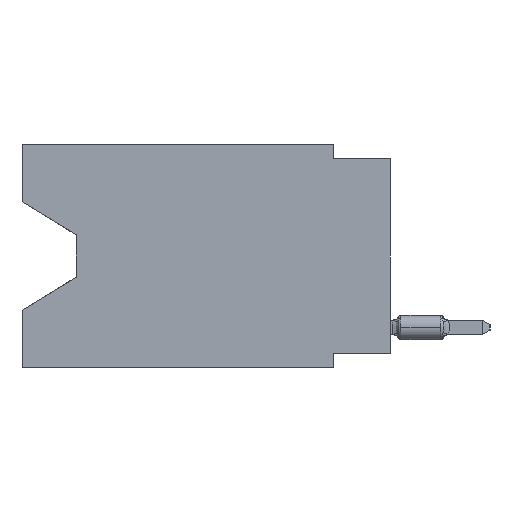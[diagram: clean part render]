
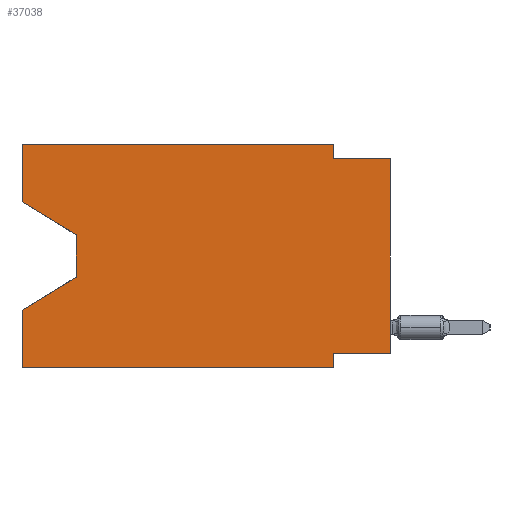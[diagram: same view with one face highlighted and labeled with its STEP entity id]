
A CAD part, left-side view. The second image highlights one B-rep face of the part: STEP entity #37038.
In plain terms, the highlighted planar face has unit normal (-1, 0, 0).
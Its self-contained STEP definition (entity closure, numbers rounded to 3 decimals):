
#512 = ORIENTED_EDGE ( 'NONE', *, *, #45183, .F. ) ;
#1542 = VERTEX_POINT ( 'NONE', #19705 ) ;
#1702 = ORIENTED_EDGE ( 'NONE', *, *, #9855, .F. ) ;
#1965 = DIRECTION ( 'NONE',  ( 0., -1., 0. ) ) ;
#3169 = LINE ( 'NONE', #44789, #12283 ) ;
#3433 = LINE ( 'NONE', #13735, #21825 ) ;
#4219 = EDGE_CURVE ( 'NONE', #1542, #48307, #7832, .T. ) ;
#4228 = CARTESIAN_POINT ( 'NONE',  ( 0., 16.383, -7.36 ) ) ;
#4435 = DIRECTION ( 'NONE',  ( 0., 0., -1. ) ) ;
#4763 = DIRECTION ( 'NONE',  ( 0., 0., -1. ) ) ;
#4885 = DIRECTION ( 'NONE',  ( 0., 0., -1. ) ) ;
#5386 = LINE ( 'NONE', #24705, #18495 ) ;
#5773 = LINE ( 'NONE', #24849, #22606 ) ;
#7021 = CARTESIAN_POINT ( 'NONE',  ( 0., 16.383, 0. ) ) ;
#7832 = LINE ( 'NONE', #16144, #19713 ) ;
#8362 = ORIENTED_EDGE ( 'NONE', *, *, #4219, .T. ) ;
#8756 = VERTEX_POINT ( 'NONE', #20245 ) ;
#9578 = EDGE_CURVE ( 'NONE', #43491, #15441, #5386, .T. ) ;
#9803 = EDGE_CURVE ( 'NONE', #30749, #11669, #10749, .T. ) ;
#9855 = EDGE_CURVE ( 'NONE', #47632, #23300, #3169, .T. ) ;
#10117 = DIRECTION ( 'NONE',  ( 0., -1., 0. ) ) ;
#10161 = EDGE_CURVE ( 'NONE', #8756, #43491, #21700, .T. ) ;
#10749 = LINE ( 'NONE', #17623, #23167 ) ;
#10930 = DIRECTION ( 'NONE',  ( 0., 0., -1. ) ) ;
#11669 = VERTEX_POINT ( 'NONE', #22764 ) ;
#12283 = VECTOR ( 'NONE', #26646, 1000. ) ;
#12544 = ORIENTED_EDGE ( 'NONE', *, *, #10161, .F. ) ;
#13652 = DIRECTION ( 'NONE',  ( 0., 0., 1. ) ) ;
#13709 = CARTESIAN_POINT ( 'NONE',  ( 0., 2.54, -9.271 ) ) ;
#13713 = EDGE_CURVE ( 'NONE', #15441, #32697, #48150, .T. ) ;
#13735 = CARTESIAN_POINT ( 'NONE',  ( 0., 0., -0.635 ) ) ;
#14557 = CARTESIAN_POINT ( 'NONE',  ( 0., 2.54, -9.906 ) ) ;
#14964 = CARTESIAN_POINT ( 'NONE',  ( 0., 0., -9.271 ) ) ;
#15086 = ORIENTED_EDGE ( 'NONE', *, *, #27840, .F. ) ;
#15441 = VERTEX_POINT ( 'NONE', #37149 ) ;
#15466 = FACE_OUTER_BOUND ( 'NONE', #23520, .T. ) ;
#15737 = LINE ( 'NONE', #30898, #34884 ) ;
#16144 = CARTESIAN_POINT ( 'NONE',  ( 0., 13.97, -4.013 ) ) ;
#16785 = AXIS2_PLACEMENT_3D ( 'NONE', #23030, #37999, #4435 ) ;
#17461 = VECTOR ( 'NONE', #34531, 1000. ) ;
#17623 = CARTESIAN_POINT ( 'NONE',  ( 0., 0., 0. ) ) ;
#17959 = ORIENTED_EDGE ( 'NONE', *, *, #21865, .F. ) ;
#18318 = CARTESIAN_POINT ( 'NONE',  ( 0., 2.54, -0.635 ) ) ;
#18495 = VECTOR ( 'NONE', #1965, 1000. ) ;
#19705 = CARTESIAN_POINT ( 'NONE',  ( 0., 13.97, -4.013 ) ) ;
#19713 = VECTOR ( 'NONE', #4885, 1000. ) ;
#20245 = CARTESIAN_POINT ( 'NONE',  ( 0., 16.383, -2.546 ) ) ;
#21497 = EDGE_CURVE ( 'NONE', #48307, #23300, #5773, .T. ) ;
#21700 = LINE ( 'NONE', #7021, #27119 ) ;
#21825 = VECTOR ( 'NONE', #47523, 1000. ) ;
#21865 = EDGE_CURVE ( 'NONE', #32697, #11669, #3433, .T. ) ;
#22606 = VECTOR ( 'NONE', #28757, 1000. ) ;
#22764 = CARTESIAN_POINT ( 'NONE',  ( 0., 0., -0.635 ) ) ;
#23030 = CARTESIAN_POINT ( 'NONE',  ( 0., 16.383, 0. ) ) ;
#23167 = VECTOR ( 'NONE', #40639, 1000. ) ;
#23300 = VERTEX_POINT ( 'NONE', #4228 ) ;
#23520 = EDGE_LOOP ( 'NONE', ( #45576, #8362, #45313, #1702, #41308, #512, #15086, #37245, #17959, #30543, #41993, #12544 ) ) ;
#23933 = LINE ( 'NONE', #42588, #17461 ) ;
#24389 = VERTEX_POINT ( 'NONE', #14557 ) ;
#24705 = CARTESIAN_POINT ( 'NONE',  ( 0., 16.383, 0. ) ) ;
#24849 = CARTESIAN_POINT ( 'NONE',  ( 0., 13.97, -5.893 ) ) ;
#26548 = EDGE_CURVE ( 'NONE', #8756, #1542, #23933, .T. ) ;
#26646 = DIRECTION ( 'NONE',  ( 0., 0., 1. ) ) ;
#26713 = PLANE ( 'NONE',  #16785 ) ;
#27119 = VECTOR ( 'NONE', #13652, 1000. ) ;
#27840 = EDGE_CURVE ( 'NONE', #30749, #31076, #15737, .T. ) ;
#28339 = CARTESIAN_POINT ( 'NONE',  ( 0., 13.97, -5.893 ) ) ;
#28757 = DIRECTION ( 'NONE',  ( 0., 0.855, -0.519 ) ) ;
#30543 = ORIENTED_EDGE ( 'NONE', *, *, #13713, .F. ) ;
#30749 = VERTEX_POINT ( 'NONE', #14964 ) ;
#30898 = CARTESIAN_POINT ( 'NONE',  ( 0., 0., -9.271 ) ) ;
#30948 = CARTESIAN_POINT ( 'NONE',  ( 0., 2.54, -9.906 ) ) ;
#31076 = VERTEX_POINT ( 'NONE', #13709 ) ;
#31426 = LINE ( 'NONE', #30948, #43567 ) ;
#32697 = VERTEX_POINT ( 'NONE', #18318 ) ;
#34531 = DIRECTION ( 'NONE',  ( 0., -0.855, -0.519 ) ) ;
#34591 = DIRECTION ( 'NONE',  ( 0., 1., 0. ) ) ;
#34884 = VECTOR ( 'NONE', #34591, 1000. ) ;
#35655 = VECTOR ( 'NONE', #10117, 1000. ) ;
#36087 = LINE ( 'NONE', #36325, #35655 ) ;
#36325 = CARTESIAN_POINT ( 'NONE',  ( 0., 16.383, -9.906 ) ) ;
#37038 = ADVANCED_FACE ( 'NONE', ( #15466 ), #26713, .F. ) ;
#37149 = CARTESIAN_POINT ( 'NONE',  ( 0., 2.54, 0. ) ) ;
#37162 = CARTESIAN_POINT ( 'NONE',  ( 0., 16.383, 0. ) ) ;
#37245 = ORIENTED_EDGE ( 'NONE', *, *, #9803, .T. ) ;
#37999 = DIRECTION ( 'NONE',  ( 1., 0., 0. ) ) ;
#40062 = CARTESIAN_POINT ( 'NONE',  ( 0., 16.383, -9.906 ) ) ;
#40639 = DIRECTION ( 'NONE',  ( 0., 0., 1. ) ) ;
#41308 = ORIENTED_EDGE ( 'NONE', *, *, #45413, .T. ) ;
#41993 = ORIENTED_EDGE ( 'NONE', *, *, #9578, .F. ) ;
#42588 = CARTESIAN_POINT ( 'NONE',  ( 0., 16.383, -2.546 ) ) ;
#43491 = VERTEX_POINT ( 'NONE', #37162 ) ;
#43567 = VECTOR ( 'NONE', #4763, 1000. ) ;
#44479 = CARTESIAN_POINT ( 'NONE',  ( 0., 2.54, 0. ) ) ;
#44789 = CARTESIAN_POINT ( 'NONE',  ( 0., 16.383, 0. ) ) ;
#45183 = EDGE_CURVE ( 'NONE', #31076, #24389, #31426, .T. ) ;
#45313 = ORIENTED_EDGE ( 'NONE', *, *, #21497, .T. ) ;
#45413 = EDGE_CURVE ( 'NONE', #47632, #24389, #36087, .T. ) ;
#45576 = ORIENTED_EDGE ( 'NONE', *, *, #26548, .T. ) ;
#46856 = VECTOR ( 'NONE', #10930, 1000. ) ;
#47523 = DIRECTION ( 'NONE',  ( 0., -1., 0. ) ) ;
#47632 = VERTEX_POINT ( 'NONE', #40062 ) ;
#48150 = LINE ( 'NONE', #44479, #46856 ) ;
#48307 = VERTEX_POINT ( 'NONE', #28339 ) ;
